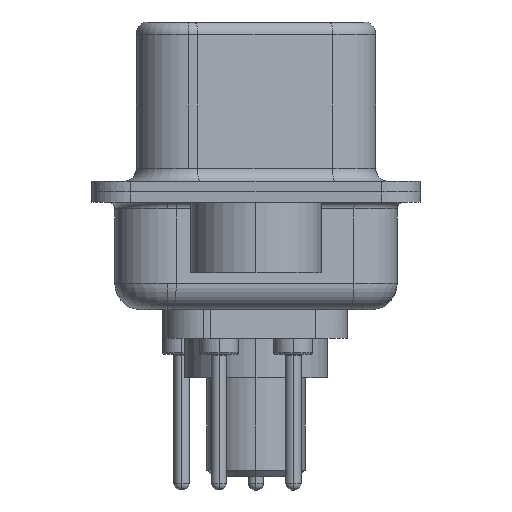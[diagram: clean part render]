
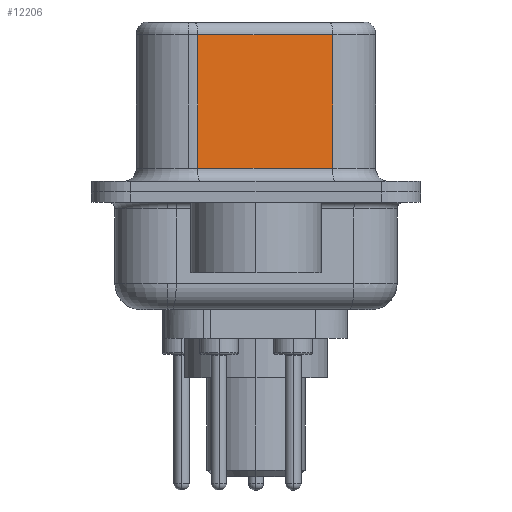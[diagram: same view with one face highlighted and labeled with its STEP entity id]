
A CAD part, left-side view. The second image highlights one B-rep face of the part: STEP entity #12206.
In plain terms, the highlighted planar face has unit normal (-0.985, -0.174, 0).
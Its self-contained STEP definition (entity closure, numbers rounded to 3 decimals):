
#149 = CARTESIAN_POINT ( 'NONE',  ( 4.585, -2.927, 6.02 ) ) ;
#189 = CARTESIAN_POINT ( 'NONE',  ( 3.675, 2.233, 6.02 ) ) ;
#608 = VERTEX_POINT ( 'NONE', #11473 ) ;
#1575 = LINE ( 'NONE', #17769, #10545 ) ;
#1780 = ORIENTED_EDGE ( 'NONE', *, *, #14052, .F. ) ;
#2190 = LINE ( 'NONE', #4153, #13900 ) ;
#2915 = VERTEX_POINT ( 'NONE', #18935 ) ;
#2970 = EDGE_LOOP ( 'NONE', ( #1780, #16701, #3598, #17590 ) ) ;
#3598 = ORIENTED_EDGE ( 'NONE', *, *, #5362, .T. ) ;
#3917 = DIRECTION ( 'NONE',  ( -0.174, 0.985, 0. ) ) ;
#3935 = DIRECTION ( 'NONE',  ( 0., 0., -1. ) ) ;
#4153 = CARTESIAN_POINT ( 'NONE',  ( 4.585, -2.927, 0.9 ) ) ;
#4846 = DIRECTION ( 'NONE',  ( -0.174, 0.985, 0. ) ) ;
#5362 = EDGE_CURVE ( 'NONE', #16666, #608, #16765, .T. ) ;
#7192 = DIRECTION ( 'NONE',  ( 0.174, -0.985, 0. ) ) ;
#7728 = LINE ( 'NONE', #149, #19687 ) ;
#10545 = VECTOR ( 'NONE', #3935, 1000. ) ;
#11473 = CARTESIAN_POINT ( 'NONE',  ( 3.675, 2.233, 0.9 ) ) ;
#11599 = EDGE_CURVE ( 'NONE', #608, #14801, #2190, .T. ) ;
#11621 = FACE_OUTER_BOUND ( 'NONE', #2970, .T. ) ;
#11825 = PLANE ( 'NONE',  #13289 ) ;
#12206 = ADVANCED_FACE ( 'NONE', ( #11621 ), #11825, .F. ) ;
#13030 = VECTOR ( 'NONE', #13935, 1000. ) ;
#13289 = AXIS2_PLACEMENT_3D ( 'NONE', #16782, #18355, #3917 ) ;
#13900 = VECTOR ( 'NONE', #7192, 1000. ) ;
#13935 = DIRECTION ( 'NONE',  ( 0., 0., -1. ) ) ;
#14052 = EDGE_CURVE ( 'NONE', #2915, #14801, #1575, .T. ) ;
#14801 = VERTEX_POINT ( 'NONE', #20141 ) ;
#16666 = VERTEX_POINT ( 'NONE', #189 ) ;
#16701 = ORIENTED_EDGE ( 'NONE', *, *, #18032, .T. ) ;
#16765 = LINE ( 'NONE', #20323, #13030 ) ;
#16782 = CARTESIAN_POINT ( 'NONE',  ( 4.585, -2.927, 6.52 ) ) ;
#17590 = ORIENTED_EDGE ( 'NONE', *, *, #11599, .T. ) ;
#17769 = CARTESIAN_POINT ( 'NONE',  ( 4.585, -2.927, 6.52 ) ) ;
#18032 = EDGE_CURVE ( 'NONE', #2915, #16666, #7728, .T. ) ;
#18355 = DIRECTION ( 'NONE',  ( 0.985, 0.174, 0. ) ) ;
#18935 = CARTESIAN_POINT ( 'NONE',  ( 4.585, -2.927, 6.02 ) ) ;
#19687 = VECTOR ( 'NONE', #4846, 1000. ) ;
#20141 = CARTESIAN_POINT ( 'NONE',  ( 4.585, -2.927, 0.9 ) ) ;
#20323 = CARTESIAN_POINT ( 'NONE',  ( 3.675, 2.233, 6.52 ) ) ;
